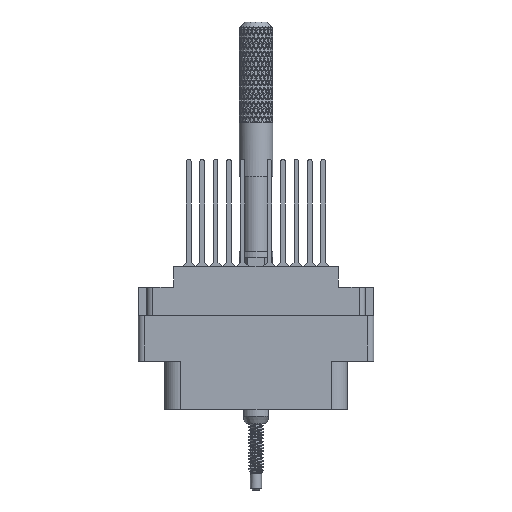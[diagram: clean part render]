
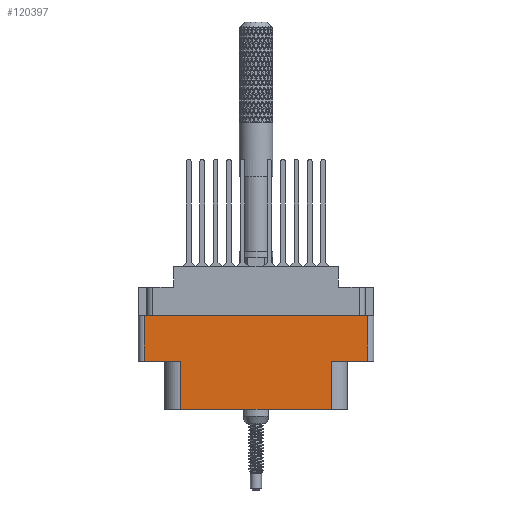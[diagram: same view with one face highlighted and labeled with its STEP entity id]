
A CAD part, front view. The second image highlights one B-rep face of the part: STEP entity #120397.
In plain terms, the highlighted planar face has unit normal (0, -1, 0).
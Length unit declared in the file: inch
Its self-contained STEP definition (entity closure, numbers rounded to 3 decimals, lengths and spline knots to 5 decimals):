
#2400 = ORIENTED_EDGE ( 'NONE', *, *, #152860, .F. ) ;
#3151 = CARTESIAN_POINT ( 'NONE',  ( 0., -0.343, -0.529 ) ) ;
#8223 = DIRECTION ( 'NONE',  ( 0., 0., 1. ) ) ;
#18663 = VECTOR ( 'NONE', #163944, 39.37008 ) ;
#25675 = ORIENTED_EDGE ( 'NONE', *, *, #60335, .T. ) ;
#26320 = ORIENTED_EDGE ( 'NONE', *, *, #130668, .T. ) ;
#27444 = VECTOR ( 'NONE', #31650, 39.37008 ) ;
#27771 = LINE ( 'NONE', #147488, #18663 ) ;
#31300 = DIRECTION ( 'NONE',  ( 0., 0., -1. ) ) ;
#31650 = DIRECTION ( 'NONE',  ( 0., 0., -1. ) ) ;
#32189 = VECTOR ( 'NONE', #31300, 39.37008 ) ;
#36197 = CARTESIAN_POINT ( 'NONE',  ( 0., -0.343, -0.274 ) ) ;
#36923 = VERTEX_POINT ( 'NONE', #46552 ) ;
#40051 = VECTOR ( 'NONE', #84860, 39.37008 ) ;
#43261 = LINE ( 'NONE', #44982, #27444 ) ;
#44982 = CARTESIAN_POINT ( 'NONE',  ( -0.624, -0.343, -0.798 ) ) ;
#46519 = PLANE ( 'NONE',  #70483 ) ;
#46552 = CARTESIAN_POINT ( 'NONE',  ( 0.42052, -0.343, -0.529 ) ) ;
#47349 = ORIENTED_EDGE ( 'NONE', *, *, #119771, .F. ) ;
#50917 = FACE_OUTER_BOUND ( 'NONE', #165306, .T. ) ;
#53287 = LINE ( 'NONE', #3151, #121301 ) ;
#56662 = VERTEX_POINT ( 'NONE', #183764 ) ;
#60335 = EDGE_CURVE ( 'NONE', #133857, #103698, #64904, .T. ) ;
#64904 = LINE ( 'NONE', #143116, #40051 ) ;
#66775 = EDGE_CURVE ( 'NONE', #56662, #133857, #143203, .T. ) ;
#70483 = AXIS2_PLACEMENT_3D ( 'NONE', #90160, #75595, #135141 ) ;
#73379 = ORIENTED_EDGE ( 'NONE', *, *, #180924, .T. ) ;
#75595 = DIRECTION ( 'NONE',  ( 0., -1., 0. ) ) ;
#84860 = DIRECTION ( 'NONE',  ( 1., 0., 0. ) ) ;
#87272 = CARTESIAN_POINT ( 'NONE',  ( -0.42052, -0.343, -0.798 ) ) ;
#88725 = VERTEX_POINT ( 'NONE', #124145 ) ;
#90160 = CARTESIAN_POINT ( 'NONE',  ( -0.656, -0.343, -0.798 ) ) ;
#90466 = VERTEX_POINT ( 'NONE', #168490 ) ;
#101947 = VERTEX_POINT ( 'NONE', #121837 ) ;
#103698 = VERTEX_POINT ( 'NONE', #123060 ) ;
#106212 = VECTOR ( 'NONE', #8223, 39.37008 ) ;
#109557 = VECTOR ( 'NONE', #172235, 39.37008 ) ;
#111184 = VERTEX_POINT ( 'NONE', #171296 ) ;
#119771 = EDGE_CURVE ( 'NONE', #111184, #36923, #53287, .T. ) ;
#120397 = ADVANCED_FACE ( 'NONE', ( #50917 ), #46519, .T. ) ;
#121301 = VECTOR ( 'NONE', #150747, 39.37008 ) ;
#121837 = CARTESIAN_POINT ( 'NONE',  ( 0.624, -0.343, -0.274 ) ) ;
#123060 = CARTESIAN_POINT ( 'NONE',  ( 0.42052, -0.343, -0.798 ) ) ;
#124145 = CARTESIAN_POINT ( 'NONE',  ( -0.624, -0.343, -0.274 ) ) ;
#124228 = DIRECTION ( 'NONE',  ( 1., 0., 0. ) ) ;
#129032 = ORIENTED_EDGE ( 'NONE', *, *, #66775, .T. ) ;
#130668 = EDGE_CURVE ( 'NONE', #111184, #101947, #140228, .T. ) ;
#133857 = VERTEX_POINT ( 'NONE', #87272 ) ;
#135141 = DIRECTION ( 'NONE',  ( 0., 0., -1. ) ) ;
#138120 = ORIENTED_EDGE ( 'NONE', *, *, #148702, .T. ) ;
#140228 = LINE ( 'NONE', #152005, #106212 ) ;
#143116 = CARTESIAN_POINT ( 'NONE',  ( -0.656, -0.343, -0.798 ) ) ;
#143203 = LINE ( 'NONE', #161161, #32189 ) ;
#147488 = CARTESIAN_POINT ( 'NONE',  ( 0., -0.343, -0.529 ) ) ;
#148324 = LINE ( 'NONE', #36197, #177768 ) ;
#148702 = EDGE_CURVE ( 'NONE', #88725, #90466, #43261, .T. ) ;
#150747 = DIRECTION ( 'NONE',  ( -1., 0., 0. ) ) ;
#152005 = CARTESIAN_POINT ( 'NONE',  ( 0.624, -0.343, -0.798 ) ) ;
#152860 = EDGE_CURVE ( 'NONE', #88725, #101947, #148324, .T. ) ;
#153446 = EDGE_CURVE ( 'NONE', #103698, #36923, #177596, .T. ) ;
#159586 = ORIENTED_EDGE ( 'NONE', *, *, #153446, .T. ) ;
#161161 = CARTESIAN_POINT ( 'NONE',  ( -0.42052, -0.343, -0.798 ) ) ;
#163944 = DIRECTION ( 'NONE',  ( 1., 0., 0. ) ) ;
#165306 = EDGE_LOOP ( 'NONE', ( #2400, #138120, #73379, #129032, #25675, #159586, #47349, #26320 ) ) ;
#168490 = CARTESIAN_POINT ( 'NONE',  ( -0.624, -0.343, -0.529 ) ) ;
#171296 = CARTESIAN_POINT ( 'NONE',  ( 0.624, -0.343, -0.529 ) ) ;
#172235 = DIRECTION ( 'NONE',  ( 0., 0., 1. ) ) ;
#172879 = CARTESIAN_POINT ( 'NONE',  ( 0.42052, -0.343, -0.529 ) ) ;
#177596 = LINE ( 'NONE', #172879, #109557 ) ;
#177768 = VECTOR ( 'NONE', #124228, 39.37008 ) ;
#180924 = EDGE_CURVE ( 'NONE', #90466, #56662, #27771, .T. ) ;
#183764 = CARTESIAN_POINT ( 'NONE',  ( -0.42052, -0.343, -0.529 ) ) ;
